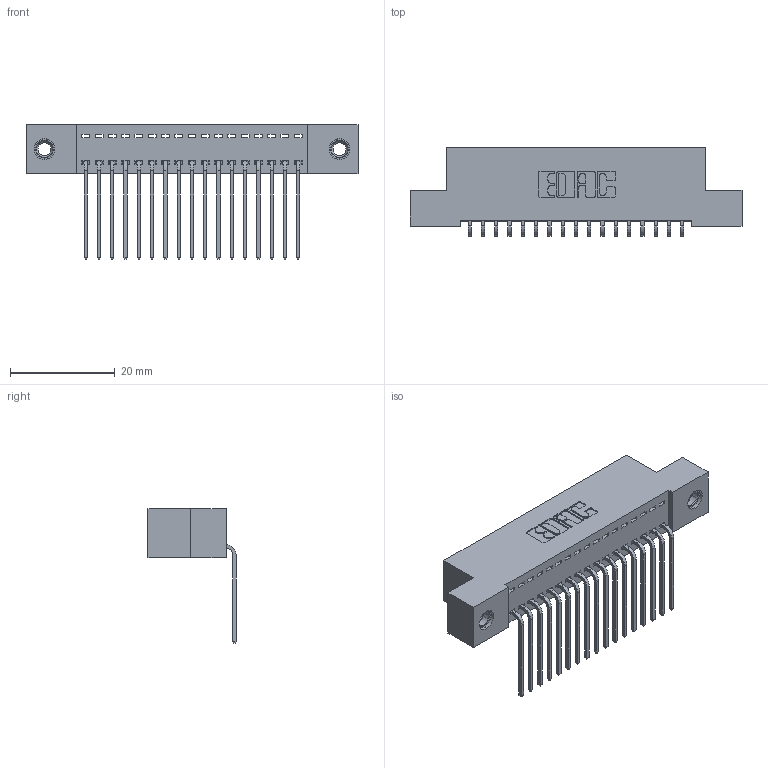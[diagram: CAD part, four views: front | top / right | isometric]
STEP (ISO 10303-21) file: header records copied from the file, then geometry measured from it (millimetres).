
FILE_DESCRIPTION (( 'STEP AP203' ), '1' );
FILE_NAME ('392-017-559-107.STEP', '2019-10-07T03:49:52', ( '' ), ( '' ), 'SwSTEP 2.0', 'SolidWorks 2016', '' );
FILE_SCHEMA (( 'CONFIG_CONTROL_DESIGN' ));
Length unit declared in the file: inch
Products named in the file (4): 342 Part_TI; 345-292-001_558 559 Tail - 1; 345-250-001_345-250-005-103; 392-017-559-107
Assembly tree (20 placements, depth 2):
  392-017-559-107
    342 Part_TI
    345-292-001_558 559 Tail - 1  x17
    345-250-001_345-250-005-103  x2
Bounding box: 63.5 x 16.83 x 25.78 mm (x, y, z)
Volume: 5519.6 mm3; surface area: 7992.3 mm2
Topology: 20 solids, 20 shells, 1190 faces, 3529 edges, 2322 vertices
Faces by surface type: plane 846, cylinder 328, cone 12, torus 4
Entity records: 14764 total; most frequent: CARTESIAN_POINT 2532, ORIENTED_EDGE 2478, DIRECTION 2219, EDGE_CURVE 1239, VECTOR 1091, LINE 1091, VERTEX_POINT 820, AXIS2_PLACEMENT_3D 564
